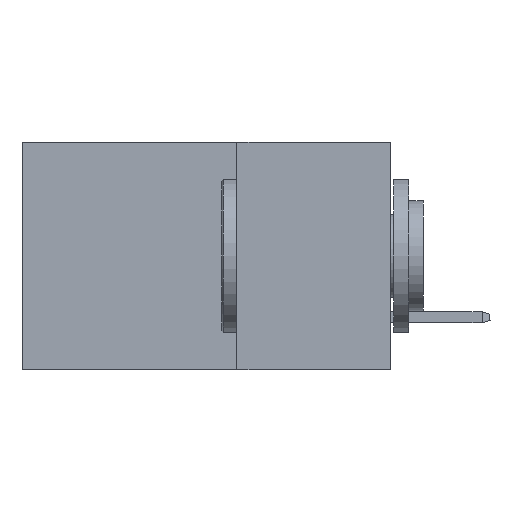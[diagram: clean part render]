
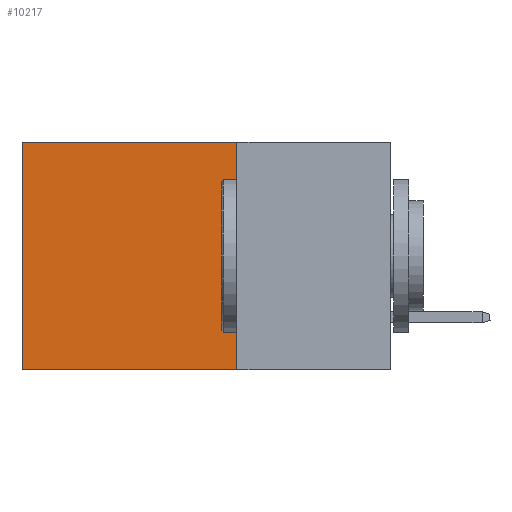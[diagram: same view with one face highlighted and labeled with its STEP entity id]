
A CAD part, left-side view. The second image highlights one B-rep face of the part: STEP entity #10217.
In plain terms, the highlighted planar face has unit normal (-1, 0, 0).
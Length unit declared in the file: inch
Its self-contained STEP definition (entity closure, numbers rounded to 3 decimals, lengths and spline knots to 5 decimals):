
#1563 = ORIENTED_EDGE ( 'NONE', *, *, #7747, .F. ) ;
#2800 = ORIENTED_EDGE ( 'NONE', *, *, #13272, .F. ) ;
#3221 = AXIS2_PLACEMENT_3D ( 'NONE', #6572, #24851, #22851 ) ;
#3279 = ORIENTED_EDGE ( 'NONE', *, *, #29289, .T. ) ;
#3838 = CARTESIAN_POINT ( 'NONE',  ( 0.2875, 0.25, -0.37 ) ) ;
#3940 = VERTEX_POINT ( 'NONE', #23338 ) ;
#4543 = VECTOR ( 'NONE', #23371, 39.37008 ) ;
#6572 = CARTESIAN_POINT ( 'NONE',  ( 0.2875, 0.25, 0. ) ) ;
#7747 = EDGE_CURVE ( 'NONE', #8904, #3940, #24915, .T. ) ;
#8208 = DIRECTION ( 'NONE',  ( 0., 1., 0. ) ) ;
#8904 = VERTEX_POINT ( 'NONE', #9561 ) ;
#9038 = CARTESIAN_POINT ( 'NONE',  ( 0.2875, 0.25, 0. ) ) ;
#9561 = CARTESIAN_POINT ( 'NONE',  ( 0.2875, 0.25, 0. ) ) ;
#9661 = VERTEX_POINT ( 'NONE', #29602 ) ;
#10115 = DIRECTION ( 'NONE',  ( 0., 0., -1. ) ) ;
#10217 = ADVANCED_FACE ( 'NONE', ( #14311 ), #20634, .F. ) ;
#10301 = LINE ( 'NONE', #21058, #4543 ) ;
#12739 = VECTOR ( 'NONE', #10115, 39.37008 ) ;
#13246 = CARTESIAN_POINT ( 'NONE',  ( 0.2875, 0.6, -0.37 ) ) ;
#13272 = EDGE_CURVE ( 'NONE', #3940, #28234, #24624, .T. ) ;
#13642 = ORIENTED_EDGE ( 'NONE', *, *, #29613, .T. ) ;
#14311 = FACE_OUTER_BOUND ( 'NONE', #18364, .T. ) ;
#15309 = VECTOR ( 'NONE', #8208, 39.37008 ) ;
#17795 = LINE ( 'NONE', #9038, #15309 ) ;
#18364 = EDGE_LOOP ( 'NONE', ( #3279, #2800, #1563, #13642 ) ) ;
#20634 = PLANE ( 'NONE',  #3221 ) ;
#21058 = CARTESIAN_POINT ( 'NONE',  ( 0.2875, 0.6, 0. ) ) ;
#22492 = VECTOR ( 'NONE', #24932, 39.37008 ) ;
#22851 = DIRECTION ( 'NONE',  ( 0., 0., -1. ) ) ;
#23338 = CARTESIAN_POINT ( 'NONE',  ( 0.2875, 0.25, -0.37 ) ) ;
#23371 = DIRECTION ( 'NONE',  ( 0., 0., -1. ) ) ;
#23558 = CARTESIAN_POINT ( 'NONE',  ( 0.2875, 0.25, 0. ) ) ;
#24624 = LINE ( 'NONE', #3838, #22492 ) ;
#24851 = DIRECTION ( 'NONE',  ( 1., 0., 0. ) ) ;
#24915 = LINE ( 'NONE', #23558, #12739 ) ;
#24932 = DIRECTION ( 'NONE',  ( 0., 1., 0. ) ) ;
#28234 = VERTEX_POINT ( 'NONE', #13246 ) ;
#29289 = EDGE_CURVE ( 'NONE', #9661, #28234, #10301, .T. ) ;
#29602 = CARTESIAN_POINT ( 'NONE',  ( 0.2875, 0.6, 0. ) ) ;
#29613 = EDGE_CURVE ( 'NONE', #8904, #9661, #17795, .T. ) ;
